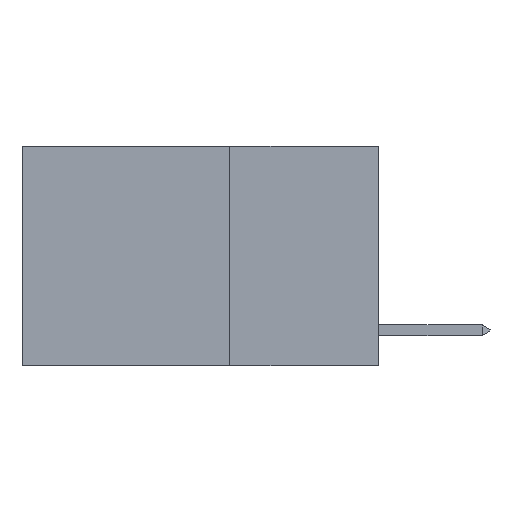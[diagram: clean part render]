
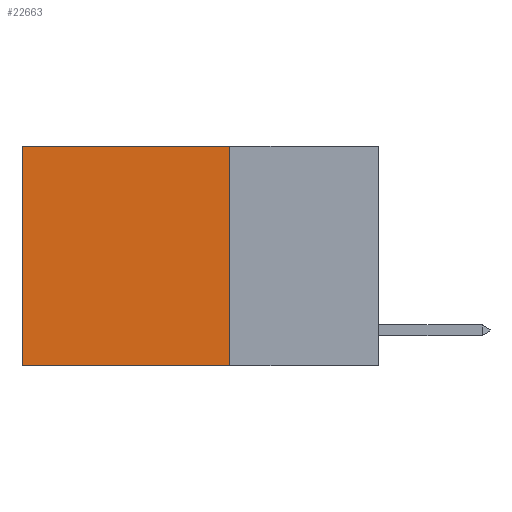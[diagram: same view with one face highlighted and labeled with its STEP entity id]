
A CAD part, left-side view. The second image highlights one B-rep face of the part: STEP entity #22663.
In plain terms, the highlighted planar face has unit normal (-1, 0, 0).
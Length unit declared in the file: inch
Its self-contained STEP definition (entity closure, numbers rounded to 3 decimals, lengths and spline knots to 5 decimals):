
#1076 = EDGE_CURVE ( 'NONE', #9165, #1279, #18496, .T. ) ;
#1279 = VERTEX_POINT ( 'NONE', #15661 ) ;
#2888 = CARTESIAN_POINT ( 'NONE',  ( 0.2625, 0.25, -0.37 ) ) ;
#3714 = VERTEX_POINT ( 'NONE', #12675 ) ;
#4060 = DIRECTION ( 'NONE',  ( 0., 0., -1. ) ) ;
#4164 = EDGE_CURVE ( 'NONE', #1279, #6284, #18059, .T. ) ;
#4478 = ORIENTED_EDGE ( 'NONE', *, *, #4164, .T. ) ;
#4628 = DIRECTION ( 'NONE',  ( 0., 1., 0. ) ) ;
#5009 = EDGE_CURVE ( 'NONE', #3714, #6284, #22737, .T. ) ;
#5319 = DIRECTION ( 'NONE',  ( 0., 0., -1. ) ) ;
#6284 = VERTEX_POINT ( 'NONE', #6513 ) ;
#6513 = CARTESIAN_POINT ( 'NONE',  ( 0.2625, 0.6, -0.37 ) ) ;
#8028 = PLANE ( 'NONE',  #10461 ) ;
#9137 = ORIENTED_EDGE ( 'NONE', *, *, #17247, .F. ) ;
#9165 = VERTEX_POINT ( 'NONE', #22720 ) ;
#9760 = VECTOR ( 'NONE', #4628, 39.37008 ) ;
#10461 = AXIS2_PLACEMENT_3D ( 'NONE', #14095, #16076, #4060 ) ;
#10657 = CARTESIAN_POINT ( 'NONE',  ( 0.2625, 0.6, 0. ) ) ;
#11422 = ORIENTED_EDGE ( 'NONE', *, *, #5009, .F. ) ;
#12003 = VECTOR ( 'NONE', #5319, 39.37008 ) ;
#12675 = CARTESIAN_POINT ( 'NONE',  ( 0.2625, 0.25, -0.37 ) ) ;
#14095 = CARTESIAN_POINT ( 'NONE',  ( 0.2625, 0.25, 0. ) ) ;
#15335 = LINE ( 'NONE', #23433, #12003 ) ;
#15661 = CARTESIAN_POINT ( 'NONE',  ( 0.2625, 0.6, 0. ) ) ;
#16076 = DIRECTION ( 'NONE',  ( 1., 0., 0. ) ) ;
#17128 = CARTESIAN_POINT ( 'NONE',  ( 0.2625, 0.25, 0. ) ) ;
#17247 = EDGE_CURVE ( 'NONE', #9165, #3714, #15335, .T. ) ;
#18059 = LINE ( 'NONE', #10657, #25116 ) ;
#18185 = FACE_OUTER_BOUND ( 'NONE', #19277, .T. ) ;
#18320 = DIRECTION ( 'NONE',  ( 0., 0., -1. ) ) ;
#18496 = LINE ( 'NONE', #17128, #23291 ) ;
#18623 = DIRECTION ( 'NONE',  ( 0., 1., 0. ) ) ;
#18842 = ORIENTED_EDGE ( 'NONE', *, *, #1076, .T. ) ;
#19277 = EDGE_LOOP ( 'NONE', ( #4478, #11422, #9137, #18842 ) ) ;
#22663 = ADVANCED_FACE ( 'NONE', ( #18185 ), #8028, .F. ) ;
#22720 = CARTESIAN_POINT ( 'NONE',  ( 0.2625, 0.25, 0. ) ) ;
#22737 = LINE ( 'NONE', #2888, #9760 ) ;
#23291 = VECTOR ( 'NONE', #18623, 39.37008 ) ;
#23433 = CARTESIAN_POINT ( 'NONE',  ( 0.2625, 0.25, 0. ) ) ;
#25116 = VECTOR ( 'NONE', #18320, 39.37008 ) ;
